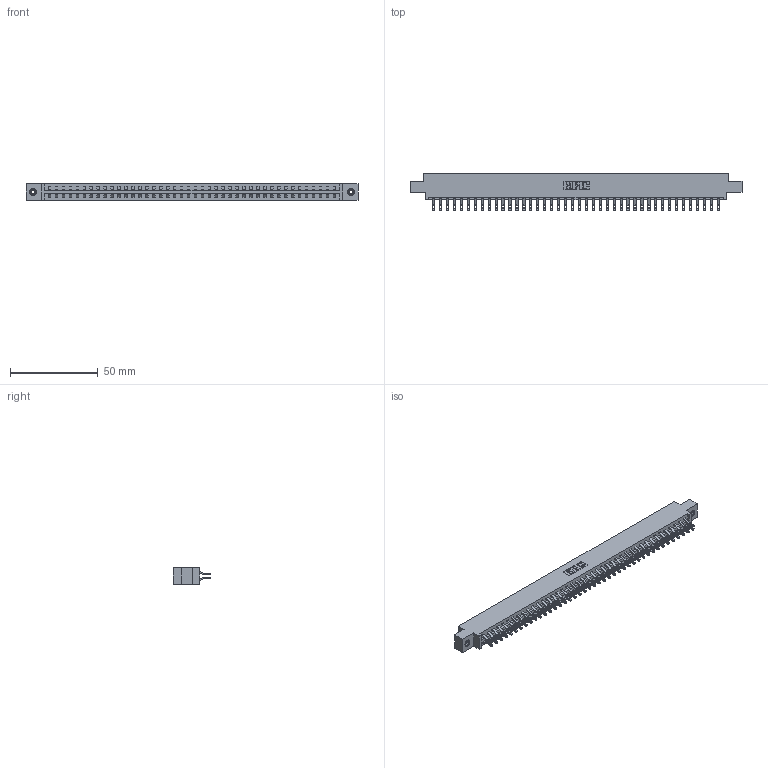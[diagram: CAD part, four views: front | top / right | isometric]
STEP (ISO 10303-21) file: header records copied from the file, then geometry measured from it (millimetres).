
FILE_DESCRIPTION (( 'STEP AP203' ), '1' );
FILE_NAME ('387-084-555-808.STEP', '2018-09-23T22:32:44', ( '' ), ( '' ), 'SwSTEP 2.0', 'SolidWorks 2016', '' );
FILE_SCHEMA (( 'CONFIG_CONTROL_DESIGN' ));
Length unit declared in the file: inch
Products named in the file (4): 345-250-001_345-250-003-102; 387-084-555-808; 337 Part_0.170 Offset - 0.156 Dia-TI; 345-292-001_555 Tail
Assembly tree (87 placements, depth 2):
  387-084-555-808
    337 Part_0.170 Offset - 0.156 Dia-TI
    345-292-001_555 Tail  x84
    345-250-001_345-250-003-102  x2
Bounding box: 189.43 x 21.47 x 9.4 mm (x, y, z)
Volume: 20083.6 mm3; surface area: 23754.5 mm2
Topology: 87 solids, 87 shells, 5218 faces, 16335 edges, 10882 vertices
Faces by surface type: plane 3130, cylinder 2072, cone 12, torus 4
Entity records: 34208 total; most frequent: CARTESIAN_POINT 5779, ORIENTED_EDGE 5678, DIRECTION 4917, EDGE_CURVE 2839, LINE 2671, VECTOR 2671, VERTEX_POINT 1888, AXIS2_PLACEMENT_3D 1123
